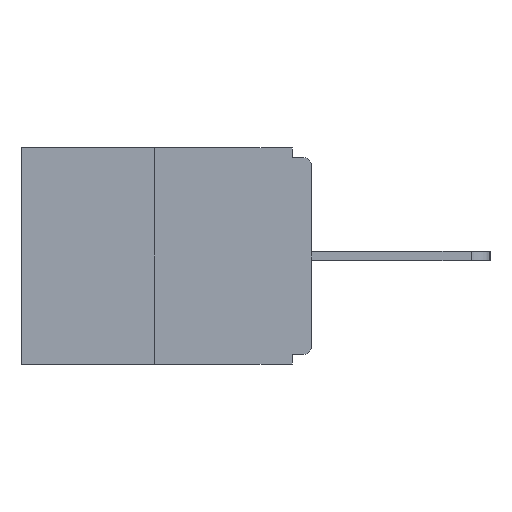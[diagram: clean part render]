
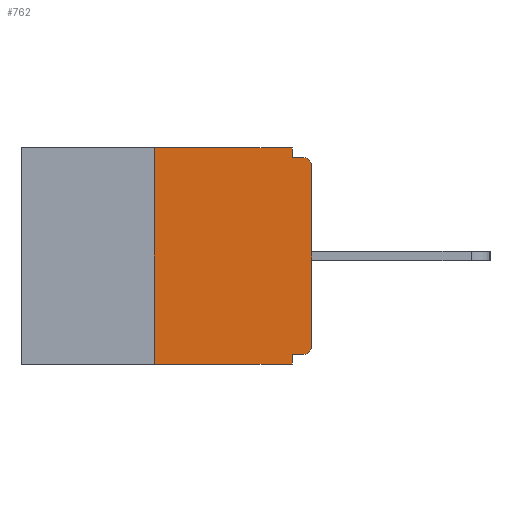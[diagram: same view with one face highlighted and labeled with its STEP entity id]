
A CAD part, left-side view. The second image highlights one B-rep face of the part: STEP entity #762.
In plain terms, the highlighted planar face has unit normal (-1, 0, 0).
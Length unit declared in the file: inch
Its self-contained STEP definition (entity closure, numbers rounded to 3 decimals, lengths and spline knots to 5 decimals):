
#57 = ORIENTED_EDGE ( 'NONE', *, *, #17315, .F. ) ;
#592 = EDGE_CURVE ( 'NONE', #20904, #25903, #20699, .T. ) ;
#714 = LINE ( 'NONE', #850, #17667 ) ;
#762 = ADVANCED_FACE ( 'NONE', ( #3318 ), #7091, .F. ) ;
#850 = CARTESIAN_POINT ( 'NONE',  ( 0., 0.031, -0.343 ) ) ;
#1096 = DIRECTION ( 'NONE',  ( 1., 0., 0. ) ) ;
#1489 = LINE ( 'NONE', #26940, #23196 ) ;
#1539 = CARTESIAN_POINT ( 'NONE',  ( 0., 0.46, 0. ) ) ;
#2073 = CARTESIAN_POINT ( 'NONE',  ( 0., 0., -0.03 ) ) ;
#2130 = VECTOR ( 'NONE', #13097, 39.37008 ) ;
#2625 = ORIENTED_EDGE ( 'NONE', *, *, #24089, .F. ) ;
#2818 = EDGE_CURVE ( 'NONE', #8088, #13608, #21825, .T. ) ;
#3060 = DIRECTION ( 'NONE',  ( 0., 0., -1. ) ) ;
#3318 = FACE_OUTER_BOUND ( 'NONE', #24664, .T. ) ;
#3803 = EDGE_CURVE ( 'NONE', #13923, #25561, #13232, .T. ) ;
#4258 = CARTESIAN_POINT ( 'NONE',  ( 0., 0.25, 0. ) ) ;
#4575 = ORIENTED_EDGE ( 'NONE', *, *, #13352, .F. ) ;
#5449 = CARTESIAN_POINT ( 'NONE',  ( 0., 0.031, 0. ) ) ;
#5650 = DIRECTION ( 'NONE',  ( 0., -1., 0. ) ) ;
#5808 = EDGE_CURVE ( 'NONE', #8151, #11831, #5899, .T. ) ;
#5899 = CIRCLE ( 'NONE', #22440, 0.015 ) ;
#5975 = ORIENTED_EDGE ( 'NONE', *, *, #2818, .T. ) ;
#6106 = CARTESIAN_POINT ( 'NONE',  ( 0., 0., -0.328 ) ) ;
#6254 = CARTESIAN_POINT ( 'NONE',  ( 0., 0.25, 0. ) ) ;
#7091 = PLANE ( 'NONE',  #19410 ) ;
#7330 = DIRECTION ( 'NONE',  ( 0., 0., -1. ) ) ;
#7488 = VERTEX_POINT ( 'NONE', #9278 ) ;
#8088 = VERTEX_POINT ( 'NONE', #2073 ) ;
#8151 = VERTEX_POINT ( 'NONE', #11273 ) ;
#8471 = LINE ( 'NONE', #6106, #18954 ) ;
#9278 = CARTESIAN_POINT ( 'NONE',  ( 0., 0.031, -0.015 ) ) ;
#9298 = CARTESIAN_POINT ( 'NONE',  ( 0., 0.46, -0.343 ) ) ;
#10416 = ORIENTED_EDGE ( 'NONE', *, *, #5808, .T. ) ;
#11108 = CARTESIAN_POINT ( 'NONE',  ( 0., 0.031, 0. ) ) ;
#11197 = DIRECTION ( 'NONE',  ( 0., 0., -1. ) ) ;
#11273 = CARTESIAN_POINT ( 'NONE',  ( 0., 0.015, -0.328 ) ) ;
#11388 = CARTESIAN_POINT ( 'NONE',  ( 0., 0.015, -0.313 ) ) ;
#11645 = EDGE_CURVE ( 'NONE', #11831, #8088, #1489, .T. ) ;
#11831 = VERTEX_POINT ( 'NONE', #26346 ) ;
#11986 = CARTESIAN_POINT ( 'NONE',  ( 0., 0.031, -0.328 ) ) ;
#12343 = LINE ( 'NONE', #22849, #15395 ) ;
#12488 = LINE ( 'NONE', #4258, #20921 ) ;
#12645 = ORIENTED_EDGE ( 'NONE', *, *, #592, .F. ) ;
#13097 = DIRECTION ( 'NONE',  ( 0., -1., 0. ) ) ;
#13232 = LINE ( 'NONE', #9298, #2130 ) ;
#13320 = AXIS2_PLACEMENT_3D ( 'NONE', #21851, #21708, #11197 ) ;
#13352 = EDGE_CURVE ( 'NONE', #25903, #7488, #20142, .T. ) ;
#13608 = VERTEX_POINT ( 'NONE', #14646 ) ;
#13923 = VERTEX_POINT ( 'NONE', #27595 ) ;
#14646 = CARTESIAN_POINT ( 'NONE',  ( 0., 0.015, -0.015 ) ) ;
#14841 = ORIENTED_EDGE ( 'NONE', *, *, #18470, .F. ) ;
#15395 = VECTOR ( 'NONE', #5650, 39.37008 ) ;
#15639 = ORIENTED_EDGE ( 'NONE', *, *, #3803, .T. ) ;
#15910 = DIRECTION ( 'NONE',  ( 0., 0., -1. ) ) ;
#16420 = ORIENTED_EDGE ( 'NONE', *, *, #11645, .T. ) ;
#17315 = EDGE_CURVE ( 'NONE', #8151, #20797, #8471, .T. ) ;
#17667 = VECTOR ( 'NONE', #24344, 39.37008 ) ;
#18021 = CARTESIAN_POINT ( 'NONE',  ( 0., 0.031, -0.343 ) ) ;
#18470 = EDGE_CURVE ( 'NONE', #20797, #25561, #714, .T. ) ;
#18954 = VECTOR ( 'NONE', #27365, 39.37008 ) ;
#19410 = AXIS2_PLACEMENT_3D ( 'NONE', #22491, #1096, #15910 ) ;
#19743 = VECTOR ( 'NONE', #3060, 39.37008 ) ;
#20142 = LINE ( 'NONE', #5449, #19743 ) ;
#20699 = LINE ( 'NONE', #1539, #26549 ) ;
#20797 = VERTEX_POINT ( 'NONE', #11986 ) ;
#20904 = VERTEX_POINT ( 'NONE', #6254 ) ;
#20921 = VECTOR ( 'NONE', #21043, 39.37008 ) ;
#21043 = DIRECTION ( 'NONE',  ( 0., 0., 1. ) ) ;
#21517 = EDGE_CURVE ( 'NONE', #13923, #20904, #12488, .T. ) ;
#21708 = DIRECTION ( 'NONE',  ( -1., 0., 0. ) ) ;
#21825 = CIRCLE ( 'NONE', #13320, 0.015 ) ;
#21851 = CARTESIAN_POINT ( 'NONE',  ( 0., 0.015, -0.03 ) ) ;
#22440 = AXIS2_PLACEMENT_3D ( 'NONE', #11388, #26080, #7330 ) ;
#22491 = CARTESIAN_POINT ( 'NONE',  ( 0., 0.46, 0. ) ) ;
#22773 = ORIENTED_EDGE ( 'NONE', *, *, #21517, .F. ) ;
#22849 = CARTESIAN_POINT ( 'NONE',  ( 0., 0., -0.015 ) ) ;
#23196 = VECTOR ( 'NONE', #24979, 39.37008 ) ;
#24089 = EDGE_CURVE ( 'NONE', #7488, #13608, #12343, .T. ) ;
#24344 = DIRECTION ( 'NONE',  ( 0., 0., -1. ) ) ;
#24664 = EDGE_LOOP ( 'NONE', ( #12645, #22773, #15639, #14841, #57, #10416, #16420, #5975, #2625, #4575 ) ) ;
#24979 = DIRECTION ( 'NONE',  ( 0., 0., 1. ) ) ;
#25561 = VERTEX_POINT ( 'NONE', #18021 ) ;
#25903 = VERTEX_POINT ( 'NONE', #11108 ) ;
#26080 = DIRECTION ( 'NONE',  ( -1., 0., 0. ) ) ;
#26346 = CARTESIAN_POINT ( 'NONE',  ( 0., 0., -0.313 ) ) ;
#26549 = VECTOR ( 'NONE', #27539, 39.37008 ) ;
#26940 = CARTESIAN_POINT ( 'NONE',  ( 0., 0., 0. ) ) ;
#27365 = DIRECTION ( 'NONE',  ( 0., 1., 0. ) ) ;
#27539 = DIRECTION ( 'NONE',  ( 0., -1., 0. ) ) ;
#27595 = CARTESIAN_POINT ( 'NONE',  ( 0., 0.25, -0.343 ) ) ;
